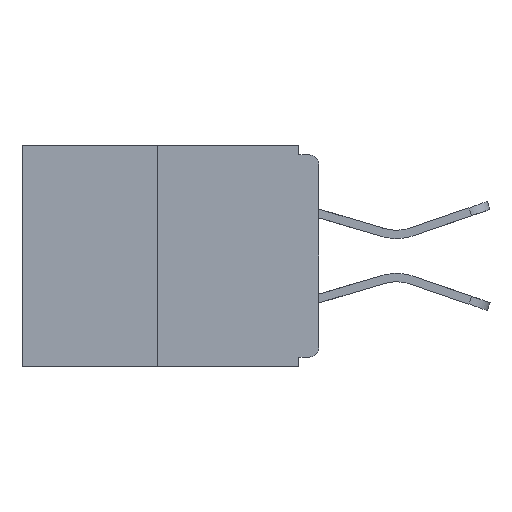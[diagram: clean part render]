
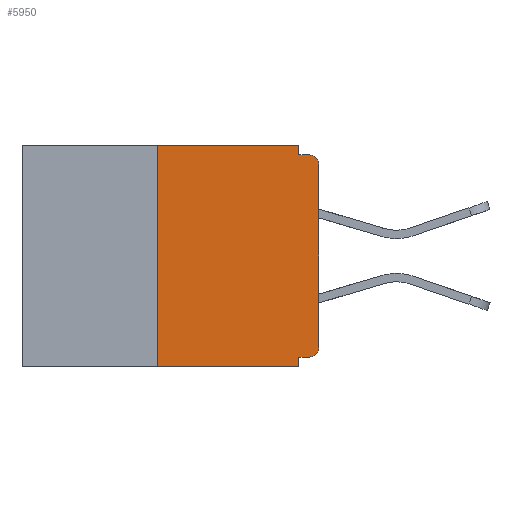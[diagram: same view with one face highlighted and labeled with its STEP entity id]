
A CAD part, left-side view. The second image highlights one B-rep face of the part: STEP entity #5950.
In plain terms, the highlighted planar face has unit normal (-1, 0, 0).
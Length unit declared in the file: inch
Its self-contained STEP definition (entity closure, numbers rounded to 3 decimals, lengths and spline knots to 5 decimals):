
#552 = CARTESIAN_POINT ( 'NONE',  ( 0., 0.031, 0. ) ) ;
#858 = EDGE_CURVE ( 'NONE', #9483, #8297, #1085, .T. ) ;
#921 = DIRECTION ( 'NONE',  ( -1., 0., 0. ) ) ;
#956 = DIRECTION ( 'NONE',  ( 0., 0., 1. ) ) ;
#1014 = EDGE_CURVE ( 'NONE', #10985, #8445, #6244, .T. ) ;
#1085 = LINE ( 'NONE', #14045, #1306 ) ;
#1306 = VECTOR ( 'NONE', #15682, 39.37008 ) ;
#1403 = DIRECTION ( 'NONE',  ( 0., 0., 1. ) ) ;
#2052 = AXIS2_PLACEMENT_3D ( 'NONE', #7942, #10890, #18447 ) ;
#2860 = ORIENTED_EDGE ( 'NONE', *, *, #15873, .T. ) ;
#3450 = VECTOR ( 'NONE', #3657, 39.37008 ) ;
#3657 = DIRECTION ( 'NONE',  ( 0., -1., 0. ) ) ;
#3675 = VECTOR ( 'NONE', #1403, 39.37008 ) ;
#3715 = VECTOR ( 'NONE', #17716, 39.37008 ) ;
#4114 = CARTESIAN_POINT ( 'NONE',  ( 0., 0., 0. ) ) ;
#4330 = DIRECTION ( 'NONE',  ( 1., 0., 0. ) ) ;
#4377 = LINE ( 'NONE', #9583, #3450 ) ;
#4470 = FACE_OUTER_BOUND ( 'NONE', #14507, .T. ) ;
#4590 = DIRECTION ( 'NONE',  ( 0., 0., -1. ) ) ;
#4885 = AXIS2_PLACEMENT_3D ( 'NONE', #14586, #921, #15954 ) ;
#4939 = ORIENTED_EDGE ( 'NONE', *, *, #9443, .T. ) ;
#5211 = CARTESIAN_POINT ( 'NONE',  ( 0., 0.031, -0.328 ) ) ;
#5348 = EDGE_CURVE ( 'NONE', #10438, #19338, #18080, .T. ) ;
#5467 = VERTEX_POINT ( 'NONE', #9463 ) ;
#5950 = ADVANCED_FACE ( 'NONE', ( #4470 ), #10586, .F. ) ;
#6244 = LINE ( 'NONE', #10152, #3675 ) ;
#6389 = CARTESIAN_POINT ( 'NONE',  ( 0., 0., -0.03 ) ) ;
#6406 = CARTESIAN_POINT ( 'NONE',  ( 0., 0., -0.313 ) ) ;
#6698 = VERTEX_POINT ( 'NONE', #6406 ) ;
#7033 = ORIENTED_EDGE ( 'NONE', *, *, #14095, .T. ) ;
#7379 = LINE ( 'NONE', #552, #14677 ) ;
#7942 = CARTESIAN_POINT ( 'NONE',  ( 0., 0.015, -0.313 ) ) ;
#8129 = CARTESIAN_POINT ( 'NONE',  ( 0., 0., -0.328 ) ) ;
#8177 = EDGE_CURVE ( 'NONE', #8445, #5467, #4377, .T. ) ;
#8243 = VECTOR ( 'NONE', #956, 39.37008 ) ;
#8297 = VERTEX_POINT ( 'NONE', #11434 ) ;
#8445 = VERTEX_POINT ( 'NONE', #13285 ) ;
#8722 = VERTEX_POINT ( 'NONE', #13570 ) ;
#8803 = LINE ( 'NONE', #17126, #15371 ) ;
#8955 = CARTESIAN_POINT ( 'NONE',  ( 0., 0.031, -0.015 ) ) ;
#9443 = EDGE_CURVE ( 'NONE', #10985, #8297, #8803, .T. ) ;
#9463 = CARTESIAN_POINT ( 'NONE',  ( 0., 0.031, 0. ) ) ;
#9483 = VERTEX_POINT ( 'NONE', #5211 ) ;
#9583 = CARTESIAN_POINT ( 'NONE',  ( 0., 0.46, 0. ) ) ;
#10152 = CARTESIAN_POINT ( 'NONE',  ( 0., 0.25, 0. ) ) ;
#10438 = VERTEX_POINT ( 'NONE', #8955 ) ;
#10490 = ORIENTED_EDGE ( 'NONE', *, *, #11091, .T. ) ;
#10586 = PLANE ( 'NONE',  #15907 ) ;
#10890 = DIRECTION ( 'NONE',  ( -1., 0., 0. ) ) ;
#10985 = VERTEX_POINT ( 'NONE', #15724 ) ;
#11091 = EDGE_CURVE ( 'NONE', #19403, #19338, #17242, .T. ) ;
#11153 = DIRECTION ( 'NONE',  ( 0., -1., 0. ) ) ;
#11408 = ORIENTED_EDGE ( 'NONE', *, *, #11932, .F. ) ;
#11434 = CARTESIAN_POINT ( 'NONE',  ( 0., 0.031, -0.343 ) ) ;
#11932 = EDGE_CURVE ( 'NONE', #5467, #10438, #7379, .T. ) ;
#12193 = LINE ( 'NONE', #4114, #8243 ) ;
#12904 = CARTESIAN_POINT ( 'NONE',  ( 0., 0., -0.015 ) ) ;
#13285 = CARTESIAN_POINT ( 'NONE',  ( 0., 0.25, 0. ) ) ;
#13354 = CARTESIAN_POINT ( 'NONE',  ( 0., 0.46, 0. ) ) ;
#13570 = CARTESIAN_POINT ( 'NONE',  ( 0., 0.015, -0.328 ) ) ;
#14045 = CARTESIAN_POINT ( 'NONE',  ( 0., 0.031, -0.343 ) ) ;
#14095 = EDGE_CURVE ( 'NONE', #6698, #19403, #12193, .T. ) ;
#14437 = ORIENTED_EDGE ( 'NONE', *, *, #5348, .F. ) ;
#14507 = EDGE_LOOP ( 'NONE', ( #15510, #15901, #4939, #17202, #18314, #2860, #7033, #10490, #14437, #11408 ) ) ;
#14586 = CARTESIAN_POINT ( 'NONE',  ( 0., 0.015, -0.03 ) ) ;
#14677 = VECTOR ( 'NONE', #17234, 39.37008 ) ;
#15371 = VECTOR ( 'NONE', #11153, 39.37008 ) ;
#15510 = ORIENTED_EDGE ( 'NONE', *, *, #8177, .F. ) ;
#15682 = DIRECTION ( 'NONE',  ( 0., 0., -1. ) ) ;
#15724 = CARTESIAN_POINT ( 'NONE',  ( 0., 0.25, -0.343 ) ) ;
#15862 = DIRECTION ( 'NONE',  ( 0., 1., 0. ) ) ;
#15873 = EDGE_CURVE ( 'NONE', #8722, #6698, #19417, .T. ) ;
#15901 = ORIENTED_EDGE ( 'NONE', *, *, #1014, .F. ) ;
#15907 = AXIS2_PLACEMENT_3D ( 'NONE', #13354, #4330, #4590 ) ;
#15954 = DIRECTION ( 'NONE',  ( 0., 0., -1. ) ) ;
#17057 = VECTOR ( 'NONE', #15862, 39.37008 ) ;
#17103 = EDGE_CURVE ( 'NONE', #8722, #9483, #18229, .T. ) ;
#17126 = CARTESIAN_POINT ( 'NONE',  ( 0., 0.46, -0.343 ) ) ;
#17202 = ORIENTED_EDGE ( 'NONE', *, *, #858, .F. ) ;
#17234 = DIRECTION ( 'NONE',  ( 0., 0., -1. ) ) ;
#17242 = CIRCLE ( 'NONE', #4885, 0.015 ) ;
#17716 = DIRECTION ( 'NONE',  ( 0., -1., 0. ) ) ;
#17865 = CARTESIAN_POINT ( 'NONE',  ( 0., 0.015, -0.015 ) ) ;
#18080 = LINE ( 'NONE', #12904, #3715 ) ;
#18229 = LINE ( 'NONE', #8129, #17057 ) ;
#18314 = ORIENTED_EDGE ( 'NONE', *, *, #17103, .F. ) ;
#18447 = DIRECTION ( 'NONE',  ( 0., 0., -1. ) ) ;
#19338 = VERTEX_POINT ( 'NONE', #17865 ) ;
#19403 = VERTEX_POINT ( 'NONE', #6389 ) ;
#19417 = CIRCLE ( 'NONE', #2052, 0.015 ) ;
